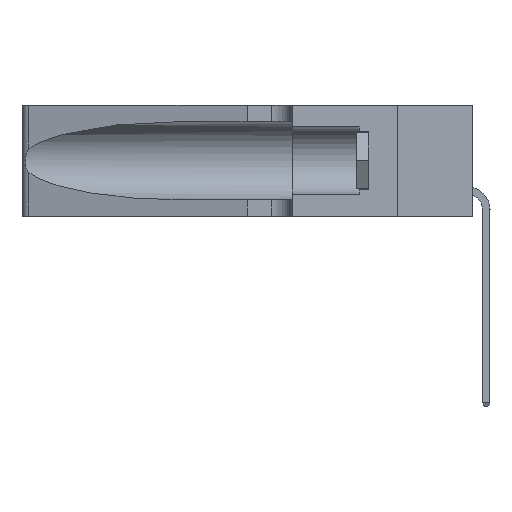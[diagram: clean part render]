
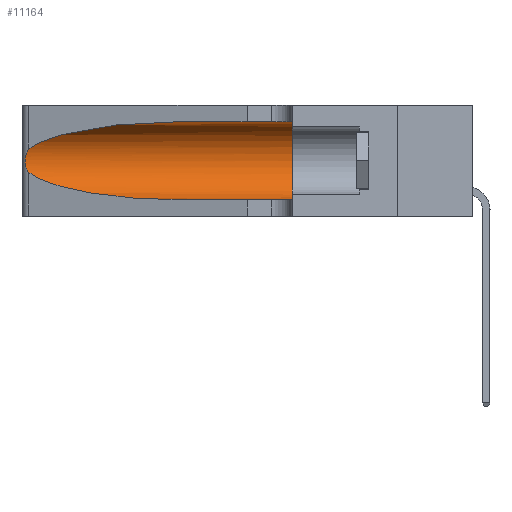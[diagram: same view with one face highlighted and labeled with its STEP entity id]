
A CAD part, left-side view. The second image highlights one B-rep face of the part: STEP entity #11164.
In plain terms, the highlighted cylindrical face has radius 3.308 mm (diameter 6.617 mm), a partial arc.
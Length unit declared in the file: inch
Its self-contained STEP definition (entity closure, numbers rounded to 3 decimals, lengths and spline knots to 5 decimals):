
#1571 = CIRCLE ( 'NONE', #17451, 0.13025 ) ;
#1894 = VERTEX_POINT ( 'NONE', #47258 ) ;
#3248 = CARTESIAN_POINT ( 'NONE',  ( 0.25555, 1.22993, 0.14849 ) ) ;
#6421 = CARTESIAN_POINT ( 'NONE',  ( 0.26017, 1.23833, 0.17102 ) ) ;
#6892 = LINE ( 'NONE', #8968, #46118 ) ;
#7715 = CARTESIAN_POINT ( 'NONE',  ( 0.1305, 0.72297, 0.31525 ) ) ;
#8968 = CARTESIAN_POINT ( 'NONE',  ( 0.1305, 1.61858, 0.31525 ) ) ;
#10205 = CARTESIAN_POINT ( 'NONE',  ( 0.25856, 1.23593, 0.16098 ) ) ;
#10522 = CARTESIAN_POINT ( 'NONE',  ( 0.25487, 1.22718, 0.22369 ) ) ;
#10845 = CARTESIAN_POINT ( 'NONE',  ( 0.26018, 1.23835, 0.19895 ) ) ;
#11164 = ADVANCED_FACE ( 'NONE', ( #14370 ), #46476, .F. ) ;
#12680 = EDGE_LOOP ( 'NONE', ( #18732, #47381, #18135, #43230, #23749, #20683 ) ) ;
#13813 = CARTESIAN_POINT ( 'NONE',  ( 0.25639, 1.23186, 0.15144 ) ) ;
#13849 = EDGE_CURVE ( 'NONE', #22093, #1894, #1571, .T. ) ;
#14370 = FACE_OUTER_BOUND ( 'NONE', #12680, .T. ) ;
#15432 =( BOUNDED_CURVE ( )  B_SPLINE_CURVE ( 3, ( #40884, #17408, #25764, #17922 ),
 .UNSPECIFIED., .F., .F. ) 
 B_SPLINE_CURVE_WITH_KNOTS ( ( 4, 4 ),
 ( 1.5708, 2.84003 ),
 .UNSPECIFIED. ) 
 CURVE ( )  GEOMETRIC_REPRESENTATION_ITEM ( )  RATIONAL_B_SPLINE_CURVE ( ( 1., 0.87, 0.87, 1. ) ) 
 REPRESENTATION_ITEM ( '' )  );
#15540 = VERTEX_POINT ( 'NONE', #21538 ) ;
#15812 = CARTESIAN_POINT ( 'NONE',  ( 0.1305, 0.35, 0.31525 ) ) ;
#15961 = VECTOR ( 'NONE', #45325, 39.37008 ) ;
#16089 = EDGE_CURVE ( 'NONE', #31686, #15540, #41999, .T. ) ;
#16866 = CARTESIAN_POINT ( 'NONE',  ( 0.1305, 0.35, 0.185 ) ) ;
#16913 = EDGE_CURVE ( 'NONE', #15540, #20715, #30174, .T. ) ;
#17408 = CARTESIAN_POINT ( 'NONE',  ( 0.18966, 0.96281, 0.31525 ) ) ;
#17451 = AXIS2_PLACEMENT_3D ( 'NONE', #16866, #46989, #28051 ) ;
#17922 = CARTESIAN_POINT ( 'NONE',  ( 0.25487, 1.22718, 0.22369 ) ) ;
#18135 = ORIENTED_EDGE ( 'NONE', *, *, #16913, .T. ) ;
#18548 = CARTESIAN_POINT ( 'NONE',  ( 0.26075, 1.23896, 0.19203 ) ) ;
#18732 = ORIENTED_EDGE ( 'NONE', *, *, #46626, .T. ) ;
#20604 = CARTESIAN_POINT ( 'NONE',  ( 0.25487, 1.22718, 0.14631 ) ) ;
#20683 = ORIENTED_EDGE ( 'NONE', *, *, #43595, .F. ) ;
#20715 = VERTEX_POINT ( 'NONE', #42007 ) ;
#21128 = DIRECTION ( 'NONE',  ( 0., -1., 0. ) ) ;
#21538 = CARTESIAN_POINT ( 'NONE',  ( 0.25487, 1.22718, 0.14631 ) ) ;
#22093 = VERTEX_POINT ( 'NONE', #15812 ) ;
#22366 = CARTESIAN_POINT ( 'NONE',  ( 0.26075, 1.23896, 0.178 ) ) ;
#23749 = ORIENTED_EDGE ( 'NONE', *, *, #13849, .F. ) ;
#24806 = DIRECTION ( 'NONE',  ( 0., 0., -1. ) ) ;
#25013 = LINE ( 'NONE', #28528, #15961 ) ;
#25572 = CARTESIAN_POINT ( 'NONE',  ( 0.25639, 1.23184, 0.21858 ) ) ;
#25764 = CARTESIAN_POINT ( 'NONE',  ( 0.2373, 1.15595, 0.28018 ) ) ;
#25884 = CARTESIAN_POINT ( 'NONE',  ( 0.25854, 1.2359, 0.20912 ) ) ;
#28051 = DIRECTION ( 'NONE',  ( 0., 0., 1. ) ) ;
#28528 = CARTESIAN_POINT ( 'NONE',  ( 0.1305, 1.61858, 0.05475 ) ) ;
#30064 = CARTESIAN_POINT ( 'NONE',  ( 0.18966, 0.96281, 0.05475 ) ) ;
#30152 = CARTESIAN_POINT ( 'NONE',  ( 0.2373, 1.15595, 0.08982 ) ) ;
#30174 =( BOUNDED_CURVE ( )  B_SPLINE_CURVE ( 3, ( #48954, #30152, #30064, #43203 ),
 .UNSPECIFIED., .F., .T. ) 
 B_SPLINE_CURVE_WITH_KNOTS ( ( 4, 4 ),
 ( 3.44316, 4.71239 ),
 .UNSPECIFIED. ) 
 CURVE ( )  GEOMETRIC_REPRESENTATION_ITEM ( )  RATIONAL_B_SPLINE_CURVE ( ( 1., 0.87, 0.87, 1. ) ) 
 REPRESENTATION_ITEM ( '' )  );
#31686 = VERTEX_POINT ( 'NONE', #40784 ) ;
#31764 = CARTESIAN_POINT ( 'NONE',  ( 0.1305, 1.61858, 0.185 ) ) ;
#35195 = EDGE_CURVE ( 'NONE', #20715, #1894, #25013, .T. ) ;
#36109 = DIRECTION ( 'NONE',  ( 0., -1., 0. ) ) ;
#39632 = CARTESIAN_POINT ( 'NONE',  ( 0.25789, 1.23486, 0.15765 ) ) ;
#40784 = CARTESIAN_POINT ( 'NONE',  ( 0.25487, 1.22718, 0.22369 ) ) ;
#40884 = CARTESIAN_POINT ( 'NONE',  ( 0.1305, 0.72297, 0.31525 ) ) ;
#41017 = CARTESIAN_POINT ( 'NONE',  ( 0.25555, 1.22994, 0.2215 ) ) ;
#41598 = AXIS2_PLACEMENT_3D ( 'NONE', #31764, #21128, #24806 ) ;
#41999 = B_SPLINE_CURVE_WITH_KNOTS ( 'NONE', 3,
 ( #10522, #41017, #25572, #44846, #25884, #10845, #18548, #22366, #6421, #10205, #39632, #13813, #3248, #20604 ),
 .UNSPECIFIED., .F., .F.,
 ( 4, 2, 2, 2, 2, 2, 4 ),
 ( 0., 0.00027, 0.00053, 0.00107, 0.0016, 0.00187, 0.00214 ),
 .UNSPECIFIED. ) ;
#42007 = CARTESIAN_POINT ( 'NONE',  ( 0.1305, 0.72297, 0.05475 ) ) ;
#42473 = VERTEX_POINT ( 'NONE', #7715 ) ;
#43203 = CARTESIAN_POINT ( 'NONE',  ( 0.1305, 0.72297, 0.05475 ) ) ;
#43230 = ORIENTED_EDGE ( 'NONE', *, *, #35195, .T. ) ;
#43595 = EDGE_CURVE ( 'NONE', #42473, #22093, #6892, .T. ) ;
#44846 = CARTESIAN_POINT ( 'NONE',  ( 0.25787, 1.23484, 0.2124 ) ) ;
#45325 = DIRECTION ( 'NONE',  ( 0., -1., 0. ) ) ;
#46118 = VECTOR ( 'NONE', #36109, 39.37008 ) ;
#46476 = CYLINDRICAL_SURFACE ( 'NONE', #41598, 0.13025 ) ;
#46626 = EDGE_CURVE ( 'NONE', #42473, #31686, #15432, .T. ) ;
#46989 = DIRECTION ( 'NONE',  ( 0., 1., 0. ) ) ;
#47258 = CARTESIAN_POINT ( 'NONE',  ( 0.1305, 0.35, 0.05475 ) ) ;
#47381 = ORIENTED_EDGE ( 'NONE', *, *, #16089, .T. ) ;
#48954 = CARTESIAN_POINT ( 'NONE',  ( 0.25487, 1.22718, 0.14631 ) ) ;
